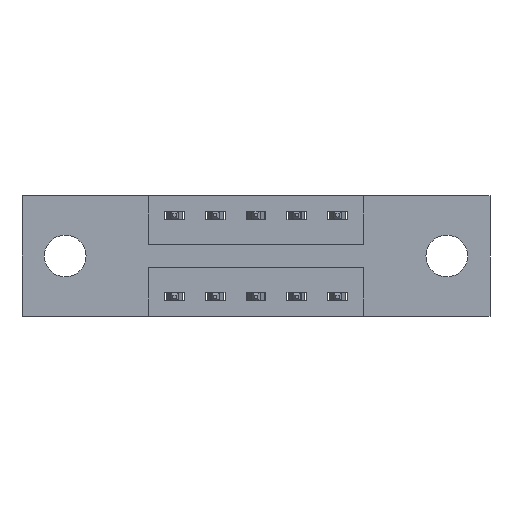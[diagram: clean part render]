
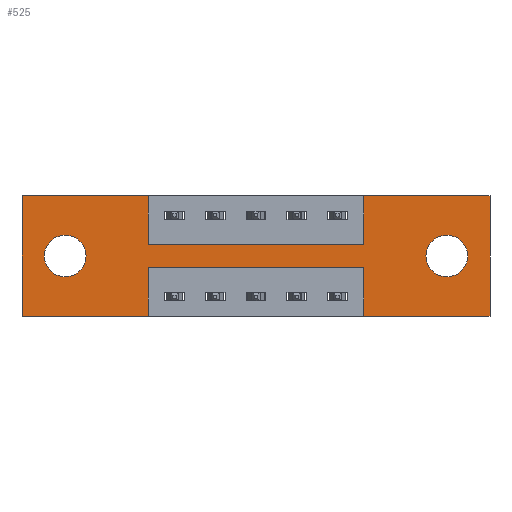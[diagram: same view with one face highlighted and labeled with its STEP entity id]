
A CAD part, front view. The second image highlights one B-rep face of the part: STEP entity #525.
In plain terms, the highlighted planar face has unit normal (0, -1, 0).
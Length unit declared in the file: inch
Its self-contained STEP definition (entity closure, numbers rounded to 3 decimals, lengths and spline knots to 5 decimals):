
#133 = DIRECTION ( 'NONE',  ( 1., 0., 0. ) ) ;
#151 = FACE_BOUND ( 'NONE', #5141, .T. ) ;
#208 = LINE ( 'NONE', #5079, #3422 ) ;
#213 = CIRCLE ( 'NONE', #8107, 0.064 ) ;
#288 = LINE ( 'NONE', #8046, #8251 ) ;
#305 = DIRECTION ( 'NONE',  ( -1., 0., 0. ) ) ;
#331 = EDGE_CURVE ( 'NONE', #4139, #551, #6006, .T. ) ;
#379 = DIRECTION ( 'NONE',  ( 0., 0., 1. ) ) ;
#390 = ORIENTED_EDGE ( 'NONE', *, *, #2686, .F. ) ;
#391 = DIRECTION ( 'NONE',  ( 0., 0., 1. ) ) ;
#525 = ADVANCED_FACE ( 'NONE', ( #6406, #151, #6575 ), #7207, .T. ) ;
#551 = VERTEX_POINT ( 'NONE', #2157 ) ;
#625 = VECTOR ( 'NONE', #1292, 39.37008 ) ;
#656 = CARTESIAN_POINT ( 'NONE',  ( 0., 0., -0.37 ) ) ;
#674 = DIRECTION ( 'NONE',  ( 0., 0., 1. ) ) ;
#738 = ORIENTED_EDGE ( 'NONE', *, *, #5482, .F. ) ;
#748 = VECTOR ( 'NONE', #3619, 39.37008 ) ;
#759 = CARTESIAN_POINT ( 'NONE',  ( 0.3875, 0., -0.15 ) ) ;
#857 = CARTESIAN_POINT ( 'NONE',  ( 1.435, 0., -0.37 ) ) ;
#1064 = CARTESIAN_POINT ( 'NONE',  ( 0., 0., -0.37 ) ) ;
#1100 = ORIENTED_EDGE ( 'NONE', *, *, #2778, .F. ) ;
#1209 = CARTESIAN_POINT ( 'NONE',  ( 0.3875, 0., 0. ) ) ;
#1221 = ORIENTED_EDGE ( 'NONE', *, *, #4494, .F. ) ;
#1252 = CARTESIAN_POINT ( 'NONE',  ( 1.3025, 0., -0.185 ) ) ;
#1292 = DIRECTION ( 'NONE',  ( -1., 0., 0. ) ) ;
#1438 = VECTOR ( 'NONE', #133, 39.37008 ) ;
#1447 = DIRECTION ( 'NONE',  ( 0., -1., 0. ) ) ;
#1454 = CARTESIAN_POINT ( 'NONE',  ( 1.3025, 0., -0.249 ) ) ;
#1587 = VERTEX_POINT ( 'NONE', #3371 ) ;
#1944 = ORIENTED_EDGE ( 'NONE', *, *, #331, .T. ) ;
#1968 = VERTEX_POINT ( 'NONE', #3579 ) ;
#1984 = EDGE_CURVE ( 'NONE', #3447, #4085, #4772, .T. ) ;
#2127 = AXIS2_PLACEMENT_3D ( 'NONE', #656, #1447, #8282 ) ;
#2157 = CARTESIAN_POINT ( 'NONE',  ( 1.3025, 0., -0.121 ) ) ;
#2242 = CARTESIAN_POINT ( 'NONE',  ( 1.0475, 0., -0.15 ) ) ;
#2342 = CARTESIAN_POINT ( 'NONE',  ( 1.0475, 0., -0.37 ) ) ;
#2362 = VERTEX_POINT ( 'NONE', #7397 ) ;
#2371 = LINE ( 'NONE', #1209, #7706 ) ;
#2388 = DIRECTION ( 'NONE',  ( 1., 0., 0. ) ) ;
#2392 = DIRECTION ( 'NONE',  ( 0., 0., 1. ) ) ;
#2633 = ORIENTED_EDGE ( 'NONE', *, *, #3208, .T. ) ;
#2686 = EDGE_CURVE ( 'NONE', #4327, #5890, #288, .T. ) ;
#2696 = CARTESIAN_POINT ( 'NONE',  ( 0.3875, 0., -0.22 ) ) ;
#2702 = CARTESIAN_POINT ( 'NONE',  ( 1.0475, 0., -0.37 ) ) ;
#2729 = CARTESIAN_POINT ( 'NONE',  ( 0.1325, 0., -0.185 ) ) ;
#2778 = EDGE_CURVE ( 'NONE', #3445, #1968, #8036, .T. ) ;
#2787 = CARTESIAN_POINT ( 'NONE',  ( 0.3875, 0., -0.37 ) ) ;
#2852 = VERTEX_POINT ( 'NONE', #2702 ) ;
#2862 = EDGE_CURVE ( 'NONE', #2362, #7898, #7655, .T. ) ;
#2869 = VERTEX_POINT ( 'NONE', #857 ) ;
#2914 = ORIENTED_EDGE ( 'NONE', *, *, #2862, .F. ) ;
#2928 = CARTESIAN_POINT ( 'NONE',  ( 1.0475, 0., 0. ) ) ;
#2969 = EDGE_CURVE ( 'NONE', #5890, #7574, #2371, .T. ) ;
#3016 = CARTESIAN_POINT ( 'NONE',  ( 0., 0., 0. ) ) ;
#3094 = EDGE_CURVE ( 'NONE', #2869, #2852, #7933, .T. ) ;
#3153 = AXIS2_PLACEMENT_3D ( 'NONE', #2729, #5019, #379 ) ;
#3208 = EDGE_CURVE ( 'NONE', #5116, #1587, #213, .T. ) ;
#3221 = EDGE_CURVE ( 'NONE', #6108, #2869, #208, .T. ) ;
#3239 = AXIS2_PLACEMENT_3D ( 'NONE', #7383, #4826, #6014 ) ;
#3371 = CARTESIAN_POINT ( 'NONE',  ( 0.1325, 0., -0.249 ) ) ;
#3422 = VECTOR ( 'NONE', #4440, 39.37008 ) ;
#3445 = VERTEX_POINT ( 'NONE', #2242 ) ;
#3447 = VERTEX_POINT ( 'NONE', #2787 ) ;
#3579 = CARTESIAN_POINT ( 'NONE',  ( 1.0475, 0., 0. ) ) ;
#3619 = DIRECTION ( 'NONE',  ( -1., 0., 0. ) ) ;
#3655 = EDGE_CURVE ( 'NONE', #1587, #5116, #7336, .T. ) ;
#3994 = EDGE_CURVE ( 'NONE', #1968, #6108, #5476, .T. ) ;
#4047 = CARTESIAN_POINT ( 'NONE',  ( 0., 0., -0.37 ) ) ;
#4085 = VERTEX_POINT ( 'NONE', #4047 ) ;
#4139 = VERTEX_POINT ( 'NONE', #1454 ) ;
#4181 = CARTESIAN_POINT ( 'NONE',  ( 1.435, 0., 0. ) ) ;
#4217 = DIRECTION ( 'NONE',  ( 1., 0., 0. ) ) ;
#4327 = VERTEX_POINT ( 'NONE', #6010 ) ;
#4406 = ORIENTED_EDGE ( 'NONE', *, *, #8226, .T. ) ;
#4408 = ORIENTED_EDGE ( 'NONE', *, *, #3221, .F. ) ;
#4440 = DIRECTION ( 'NONE',  ( 0., 0., -1. ) ) ;
#4454 = CARTESIAN_POINT ( 'NONE',  ( 0.3875, 0., -0.22 ) ) ;
#4494 = EDGE_CURVE ( 'NONE', #7574, #3445, #6380, .T. ) ;
#4499 = ORIENTED_EDGE ( 'NONE', *, *, #3994, .F. ) ;
#4549 = ORIENTED_EDGE ( 'NONE', *, *, #2969, .F. ) ;
#4642 = EDGE_CURVE ( 'NONE', #2852, #2362, #5993, .T. ) ;
#4744 = VECTOR ( 'NONE', #305, 39.37008 ) ;
#4772 = LINE ( 'NONE', #1064, #748 ) ;
#4826 = DIRECTION ( 'NONE',  ( 0., 1., 0. ) ) ;
#4930 = AXIS2_PLACEMENT_3D ( 'NONE', #1252, #6963, #7463 ) ;
#4950 = CARTESIAN_POINT ( 'NONE',  ( 0.3875, 0., -0.15 ) ) ;
#5019 = DIRECTION ( 'NONE',  ( 0., 1., 0. ) ) ;
#5079 = CARTESIAN_POINT ( 'NONE',  ( 1.435, 0., 0. ) ) ;
#5116 = VERTEX_POINT ( 'NONE', #6017 ) ;
#5141 = EDGE_LOOP ( 'NONE', ( #2633, #5387 ) ) ;
#5181 = VECTOR ( 'NONE', #5424, 39.37008 ) ;
#5387 = ORIENTED_EDGE ( 'NONE', *, *, #3655, .T. ) ;
#5424 = DIRECTION ( 'NONE',  ( 0., 0., 1. ) ) ;
#5445 = EDGE_LOOP ( 'NONE', ( #4406, #1944 ) ) ;
#5476 = LINE ( 'NONE', #3016, #6939 ) ;
#5482 = EDGE_CURVE ( 'NONE', #4085, #4327, #7562, .T. ) ;
#5820 = CARTESIAN_POINT ( 'NONE',  ( 0.3875, 0., 0. ) ) ;
#5890 = VERTEX_POINT ( 'NONE', #5820 ) ;
#5923 = DIRECTION ( 'NONE',  ( 0., 0., -1. ) ) ;
#5993 = LINE ( 'NONE', #2342, #7205 ) ;
#6006 = CIRCLE ( 'NONE', #4930, 0.064 ) ;
#6010 = CARTESIAN_POINT ( 'NONE',  ( 0., 0., 0. ) ) ;
#6014 = DIRECTION ( 'NONE',  ( 0., 0., -1. ) ) ;
#6017 = CARTESIAN_POINT ( 'NONE',  ( 0.1325, 0., -0.121 ) ) ;
#6042 = CARTESIAN_POINT ( 'NONE',  ( 0., 0., -0.37 ) ) ;
#6108 = VERTEX_POINT ( 'NONE', #4181 ) ;
#6380 = LINE ( 'NONE', #759, #1438 ) ;
#6406 = FACE_BOUND ( 'NONE', #5445, .T. ) ;
#6525 = LINE ( 'NONE', #7818, #8198 ) ;
#6553 = ORIENTED_EDGE ( 'NONE', *, *, #1984, .F. ) ;
#6575 = FACE_OUTER_BOUND ( 'NONE', #6915, .T. ) ;
#6779 = DIRECTION ( 'NONE',  ( 0., 1., 0. ) ) ;
#6822 = VECTOR ( 'NONE', #674, 39.37008 ) ;
#6865 = CIRCLE ( 'NONE', #3239, 0.064 ) ;
#6915 = EDGE_LOOP ( 'NONE', ( #7451, #2914, #7369, #7343, #4408, #4499, #1100, #1221, #4549, #390, #738, #6553 ) ) ;
#6939 = VECTOR ( 'NONE', #2388, 39.37008 ) ;
#6963 = DIRECTION ( 'NONE',  ( 0., 1., 0. ) ) ;
#7205 = VECTOR ( 'NONE', #2392, 39.37008 ) ;
#7207 = PLANE ( 'NONE',  #2127 ) ;
#7336 = CIRCLE ( 'NONE', #3153, 0.064 ) ;
#7343 = ORIENTED_EDGE ( 'NONE', *, *, #3094, .F. ) ;
#7369 = ORIENTED_EDGE ( 'NONE', *, *, #4642, .F. ) ;
#7382 = EDGE_CURVE ( 'NONE', #7898, #3447, #6525, .T. ) ;
#7383 = CARTESIAN_POINT ( 'NONE',  ( 1.3025, 0., -0.185 ) ) ;
#7397 = CARTESIAN_POINT ( 'NONE',  ( 1.0475, 0., -0.22 ) ) ;
#7451 = ORIENTED_EDGE ( 'NONE', *, *, #7382, .F. ) ;
#7463 = DIRECTION ( 'NONE',  ( 0., 0., -1. ) ) ;
#7562 = LINE ( 'NONE', #8256, #6822 ) ;
#7574 = VERTEX_POINT ( 'NONE', #4950 ) ;
#7655 = LINE ( 'NONE', #4454, #625 ) ;
#7706 = VECTOR ( 'NONE', #8188, 39.37008 ) ;
#7818 = CARTESIAN_POINT ( 'NONE',  ( 0.3875, 0., -0.37 ) ) ;
#7898 = VERTEX_POINT ( 'NONE', #2696 ) ;
#7933 = LINE ( 'NONE', #6042, #4744 ) ;
#8036 = LINE ( 'NONE', #2928, #5181 ) ;
#8046 = CARTESIAN_POINT ( 'NONE',  ( 0., 0., 0. ) ) ;
#8107 = AXIS2_PLACEMENT_3D ( 'NONE', #8180, #6779, #391 ) ;
#8180 = CARTESIAN_POINT ( 'NONE',  ( 0.1325, 0., -0.185 ) ) ;
#8188 = DIRECTION ( 'NONE',  ( 0., 0., -1. ) ) ;
#8198 = VECTOR ( 'NONE', #5923, 39.37008 ) ;
#8226 = EDGE_CURVE ( 'NONE', #551, #4139, #6865, .T. ) ;
#8251 = VECTOR ( 'NONE', #4217, 39.37008 ) ;
#8256 = CARTESIAN_POINT ( 'NONE',  ( 0., 0., 0. ) ) ;
#8282 = DIRECTION ( 'NONE',  ( 0., 0., -1. ) ) ;
